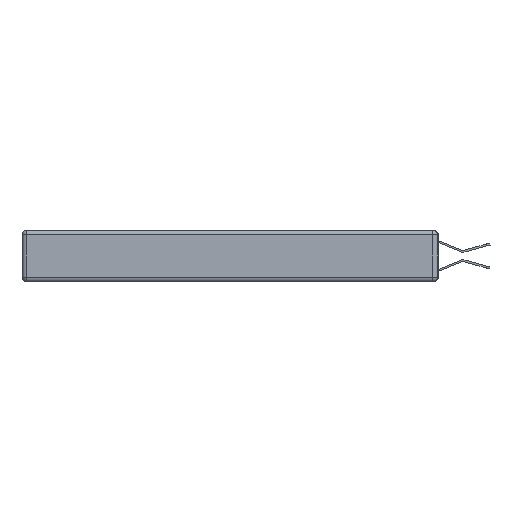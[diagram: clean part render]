
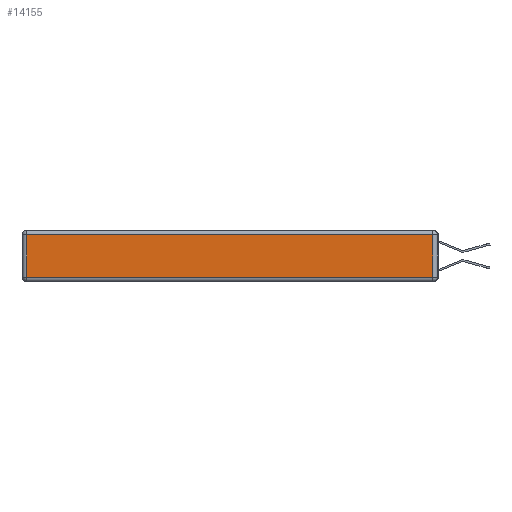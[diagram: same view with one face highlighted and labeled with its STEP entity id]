
A CAD part, left-side view. The second image highlights one B-rep face of the part: STEP entity #14155.
In plain terms, the highlighted planar face has unit normal (-1, 0, 0).
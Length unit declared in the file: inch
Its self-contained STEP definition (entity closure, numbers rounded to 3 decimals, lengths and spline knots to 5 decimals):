
#175 = VERTEX_POINT ( 'NONE', #3026 ) ;
#919 = DIRECTION ( 'NONE',  ( 0., 0., 1. ) ) ;
#1063 = LINE ( 'NONE', #1301, #7531 ) ;
#1301 = CARTESIAN_POINT ( 'NONE',  ( 0., 2.72, -0.343 ) ) ;
#2731 = EDGE_LOOP ( 'NONE', ( #9371, #3698, #10287, #8547 ) ) ;
#2906 = DIRECTION ( 'NONE',  ( 0., -1., 0. ) ) ;
#3026 = CARTESIAN_POINT ( 'NONE',  ( 0., 0.03, -0.03 ) ) ;
#3698 = ORIENTED_EDGE ( 'NONE', *, *, #10319, .T. ) ;
#4137 = DIRECTION ( 'NONE',  ( 0., 1., 0. ) ) ;
#5571 = EDGE_CURVE ( 'NONE', #19628, #12071, #1063, .T. ) ;
#6005 = FACE_OUTER_BOUND ( 'NONE', #2731, .T. ) ;
#6091 = CARTESIAN_POINT ( 'NONE',  ( 0., 2.72, -0.313 ) ) ;
#6562 = LINE ( 'NONE', #20879, #10957 ) ;
#7531 = VECTOR ( 'NONE', #10419, 39.37008 ) ;
#7682 = LINE ( 'NONE', #13138, #13998 ) ;
#8547 = ORIENTED_EDGE ( 'NONE', *, *, #5571, .T. ) ;
#9371 = ORIENTED_EDGE ( 'NONE', *, *, #12846, .T. ) ;
#9413 = VERTEX_POINT ( 'NONE', #17207 ) ;
#10287 = ORIENTED_EDGE ( 'NONE', *, *, #21378, .T. ) ;
#10319 = EDGE_CURVE ( 'NONE', #9413, #175, #13351, .T. ) ;
#10419 = DIRECTION ( 'NONE',  ( 0., 0., -1. ) ) ;
#10957 = VECTOR ( 'NONE', #2906, 39.37008 ) ;
#11465 = DIRECTION ( 'NONE',  ( -1., 0., 0. ) ) ;
#12071 = VERTEX_POINT ( 'NONE', #6091 ) ;
#12846 = EDGE_CURVE ( 'NONE', #12071, #9413, #6562, .T. ) ;
#13138 = CARTESIAN_POINT ( 'NONE',  ( 0., 2.75, -0.03 ) ) ;
#13235 = PLANE ( 'NONE',  #15876 ) ;
#13351 = LINE ( 'NONE', #22344, #22221 ) ;
#13998 = VECTOR ( 'NONE', #4137, 39.37008 ) ;
#14155 = ADVANCED_FACE ( 'NONE', ( #6005 ), #13235, .T. ) ;
#15876 = AXIS2_PLACEMENT_3D ( 'NONE', #20446, #11465, #16898 ) ;
#16898 = DIRECTION ( 'NONE',  ( 0., 0., 1. ) ) ;
#17073 = CARTESIAN_POINT ( 'NONE',  ( 0., 2.72, -0.03 ) ) ;
#17207 = CARTESIAN_POINT ( 'NONE',  ( 0., 0.03, -0.313 ) ) ;
#19628 = VERTEX_POINT ( 'NONE', #17073 ) ;
#20446 = CARTESIAN_POINT ( 'NONE',  ( 0., 0., -0.343 ) ) ;
#20879 = CARTESIAN_POINT ( 'NONE',  ( 0., 0., -0.313 ) ) ;
#21378 = EDGE_CURVE ( 'NONE', #175, #19628, #7682, .T. ) ;
#22221 = VECTOR ( 'NONE', #919, 39.37008 ) ;
#22344 = CARTESIAN_POINT ( 'NONE',  ( 0., 0.03, -0.343 ) ) ;
